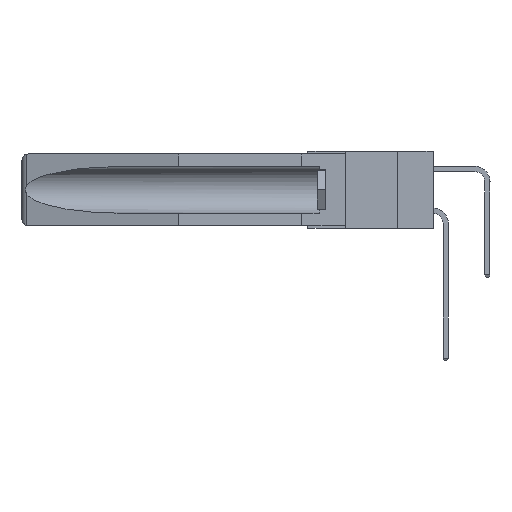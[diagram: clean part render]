
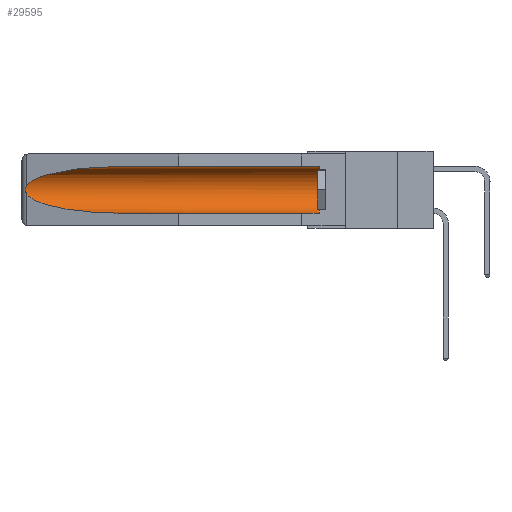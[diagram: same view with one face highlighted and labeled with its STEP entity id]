
A CAD part, left-side view. The second image highlights one B-rep face of the part: STEP entity #29595.
In plain terms, the highlighted cylindrical face has radius 2.857 mm (diameter 5.715 mm), a partial arc.
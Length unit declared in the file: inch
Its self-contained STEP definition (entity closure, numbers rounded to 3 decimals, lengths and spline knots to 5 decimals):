
#44 = LINE ( 'NONE', #2398, #22446 ) ;
#170 = VERTEX_POINT ( 'NONE', #5743 ) ;
#2040 = CYLINDRICAL_SURFACE ( 'NONE', #12839, 0.1125 ) ;
#2398 = CARTESIAN_POINT ( 'NONE',  ( 0.155, -0.30754, -0.059 ) ) ;
#2592 = CARTESIAN_POINT ( 'NONE',  ( 0.2675, 1.53308, -0.16763 ) ) ;
#3096 = ORIENTED_EDGE ( 'NONE', *, *, #3315, .T. ) ;
#3315 = EDGE_CURVE ( 'NONE', #170, #3785, #9725, .T. ) ;
#3785 = VERTEX_POINT ( 'NONE', #26367 ) ;
#4033 = CARTESIAN_POINT ( 'NONE',  ( 0.155, 0.126, -0.1715 ) ) ;
#4356 = EDGE_CURVE ( 'NONE', #17395, #10196, #8473, .T. ) ;
#4497 = CARTESIAN_POINT ( 'NONE',  ( 0.155, 1.07973, -0.284 ) ) ;
#4856 = ORIENTED_EDGE ( 'NONE', *, *, #31442, .T. ) ;
#4991 = CARTESIAN_POINT ( 'NONE',  ( 0.25451, 1.48313, -0.24835 ) ) ;
#5204 = CARTESIAN_POINT ( 'NONE',  ( 0.155, 1.07973, -0.059 ) ) ;
#5743 = CARTESIAN_POINT ( 'NONE',  ( 0.155, 0.126, -0.284 ) ) ;
#5868 = CARTESIAN_POINT ( 'NONE',  ( 0.26537, 1.52718, -0.14972 ) ) ;
#5981 = VERTEX_POINT ( 'NONE', #30359 ) ;
#6265 = DIRECTION ( 'NONE',  ( 0., 1., 0. ) ) ;
#6359 =( BOUNDED_CURVE ( )  B_SPLINE_CURVE ( 3, ( #15520, #4991, #12609, #26249 ),
 .UNSPECIFIED., .F., .F. ) 
 B_SPLINE_CURVE_WITH_KNOTS ( ( 4, 4 ),
 ( 0.1948, 1.5708 ),
 .UNSPECIFIED. ) 
 CURVE ( )  GEOMETRIC_REPRESENTATION_ITEM ( )  RATIONAL_B_SPLINE_CURVE ( ( 1., 0.848, 0.848, 1. ) ) 
 REPRESENTATION_ITEM ( '' )  );
#7890 = CARTESIAN_POINT ( 'NONE',  ( 0.26597, 1.52961, -0.15275 ) ) ;
#8123 = CARTESIAN_POINT ( 'NONE',  ( 0.26597, 1.5296, -0.19026 ) ) ;
#8282 = LINE ( 'NONE', #20822, #32805 ) ;
#8473 = B_SPLINE_CURVE_WITH_KNOTS ( 'NONE', 3,
 ( #26621, #7890, #10683, #16131, #2592, #29269, #26847, #13333, #8123, #31908 ),
 .UNSPECIFIED., .F., .F.,
 ( 4, 2, 2, 2, 4 ),
 ( 0., 0.00029, 0.00058, 0.00087, 0.00117 ),
 .UNSPECIFIED. ) ;
#8760 = CARTESIAN_POINT ( 'NONE',  ( 0.155, -0.30754, -0.1715 ) ) ;
#8963 = ORIENTED_EDGE ( 'NONE', *, *, #11976, .T. ) ;
#9725 = CIRCLE ( 'NONE', #31854, 0.1125 ) ;
#10196 = VERTEX_POINT ( 'NONE', #25039 ) ;
#10683 = CARTESIAN_POINT ( 'NONE',  ( 0.26654, 1.53092, -0.15636 ) ) ;
#10746 = CARTESIAN_POINT ( 'NONE',  ( 0.25451, 1.48313, -0.09465 ) ) ;
#11976 = EDGE_CURVE ( 'NONE', #5981, #17395, #24468, .T. ) ;
#12609 = CARTESIAN_POINT ( 'NONE',  ( 0.21114, 1.30732, -0.284 ) ) ;
#12839 = AXIS2_PLACEMENT_3D ( 'NONE', #8760, #33029, #19795 ) ;
#13130 = ORIENTED_EDGE ( 'NONE', *, *, #25735, .F. ) ;
#13333 = CARTESIAN_POINT ( 'NONE',  ( 0.26655, 1.53094, -0.18657 ) ) ;
#14569 = VERTEX_POINT ( 'NONE', #4497 ) ;
#15520 = CARTESIAN_POINT ( 'NONE',  ( 0.26537, 1.52718, -0.19328 ) ) ;
#16131 = CARTESIAN_POINT ( 'NONE',  ( 0.2673, 1.5327, -0.16383 ) ) ;
#17395 = VERTEX_POINT ( 'NONE', #5868 ) ;
#18525 = CARTESIAN_POINT ( 'NONE',  ( 0.26537, 1.52718, -0.14972 ) ) ;
#19795 = DIRECTION ( 'NONE',  ( 0., 0., 1. ) ) ;
#20822 = CARTESIAN_POINT ( 'NONE',  ( 0.155, -0.30754, -0.284 ) ) ;
#22446 = VECTOR ( 'NONE', #6265, 39.37008 ) ;
#22600 = DIRECTION ( 'NONE',  ( 0., 0., 1. ) ) ;
#23624 = DIRECTION ( 'NONE',  ( 0., 1., 0. ) ) ;
#23860 = ORIENTED_EDGE ( 'NONE', *, *, #4356, .T. ) ;
#24468 =( BOUNDED_CURVE ( )  B_SPLINE_CURVE ( 3, ( #5204, #31751, #10746, #18525 ),
 .UNSPECIFIED., .F., .F. ) 
 B_SPLINE_CURVE_WITH_KNOTS ( ( 4, 4 ),
 ( 4.71239, 6.08839 ),
 .UNSPECIFIED. ) 
 CURVE ( )  GEOMETRIC_REPRESENTATION_ITEM ( )  RATIONAL_B_SPLINE_CURVE ( ( 1., 0.848, 0.848, 1. ) ) 
 REPRESENTATION_ITEM ( '' )  );
#25039 = CARTESIAN_POINT ( 'NONE',  ( 0.26537, 1.52718, -0.19328 ) ) ;
#25735 = EDGE_CURVE ( 'NONE', #170, #14569, #8282, .T. ) ;
#25776 = EDGE_CURVE ( 'NONE', #3785, #5981, #44, .T. ) ;
#26249 = CARTESIAN_POINT ( 'NONE',  ( 0.155, 1.07973, -0.284 ) ) ;
#26367 = CARTESIAN_POINT ( 'NONE',  ( 0.155, 0.126, -0.059 ) ) ;
#26621 = CARTESIAN_POINT ( 'NONE',  ( 0.26537, 1.52718, -0.14972 ) ) ;
#26847 = CARTESIAN_POINT ( 'NONE',  ( 0.2673, 1.53269, -0.17917 ) ) ;
#27767 = FACE_OUTER_BOUND ( 'NONE', #29466, .T. ) ;
#29269 = CARTESIAN_POINT ( 'NONE',  ( 0.2675, 1.53308, -0.17534 ) ) ;
#29466 = EDGE_LOOP ( 'NONE', ( #8963, #23860, #4856, #13130, #3096, #32729 ) ) ;
#29595 = ADVANCED_FACE ( 'NONE', ( #27767 ), #2040, .F. ) ;
#30359 = CARTESIAN_POINT ( 'NONE',  ( 0.155, 1.07973, -0.059 ) ) ;
#30593 = DIRECTION ( 'NONE',  ( 0., -1., 0. ) ) ;
#31442 = EDGE_CURVE ( 'NONE', #10196, #14569, #6359, .T. ) ;
#31751 = CARTESIAN_POINT ( 'NONE',  ( 0.21114, 1.30732, -0.059 ) ) ;
#31854 = AXIS2_PLACEMENT_3D ( 'NONE', #4033, #30593, #22600 ) ;
#31908 = CARTESIAN_POINT ( 'NONE',  ( 0.26537, 1.52718, -0.19328 ) ) ;
#32729 = ORIENTED_EDGE ( 'NONE', *, *, #25776, .T. ) ;
#32805 = VECTOR ( 'NONE', #23624, 39.37008 ) ;
#33029 = DIRECTION ( 'NONE',  ( 0., 1., 0. ) ) ;
